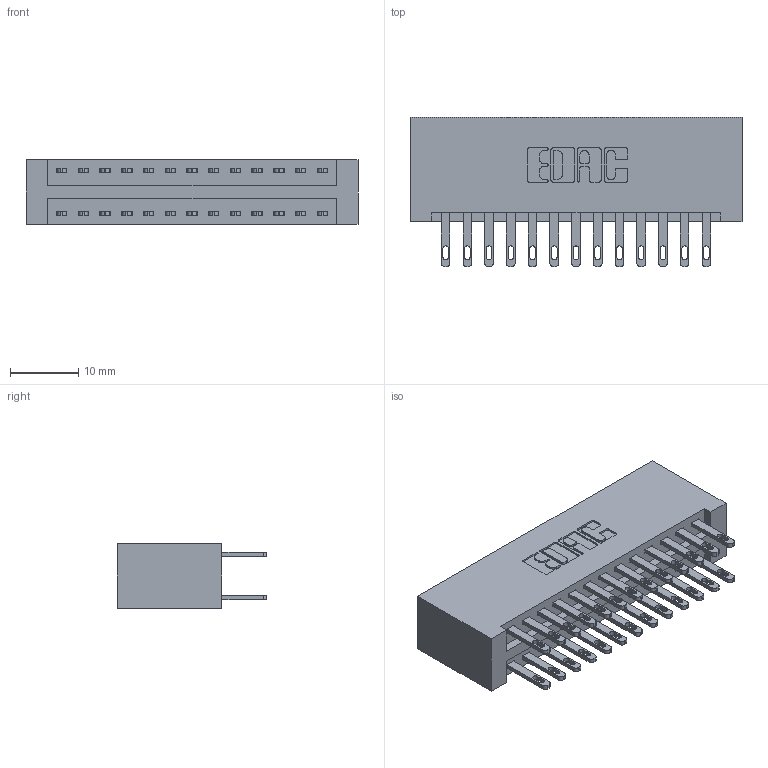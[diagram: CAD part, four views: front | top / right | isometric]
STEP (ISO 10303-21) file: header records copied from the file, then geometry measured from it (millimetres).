
FILE_DESCRIPTION (( 'STEP AP203' ), '1' );
FILE_NAME ('346-026-500-201.STEP', '2022-05-19T00:48:54', ( '' ), ( '' ), 'SwSTEP 2.0', 'SolidWorks 2020', '' );
FILE_SCHEMA (( 'CONFIG_CONTROL_DESIGN' ));
Length unit declared in the file: inch
Products named in the file (3): 345-292-001_345-293-100; 346 Part_No Mounting Lugs; 346-026-500-201
Assembly tree (27 placements, depth 2):
  346-026-500-201
    346 Part_No Mounting Lugs
    345-292-001_345-293-100  x26
Bounding box: 48.51 x 21.84 x 9.4 mm (x, y, z)
Volume: 5158.2 mm3; surface area: 7069.8 mm2
Topology: 27 solids, 27 shells, 1362 faces, 4127 edges, 2750 vertices
Faces by surface type: plane 826, cylinder 536
Entity records: 12041 total; most frequent: CARTESIAN_POINT 2020, ORIENTED_EDGE 1954, DIRECTION 1829, EDGE_CURVE 977, LINE 797, VECTOR 797, VERTEX_POINT 650, AXIS2_PLACEMENT_3D 516
